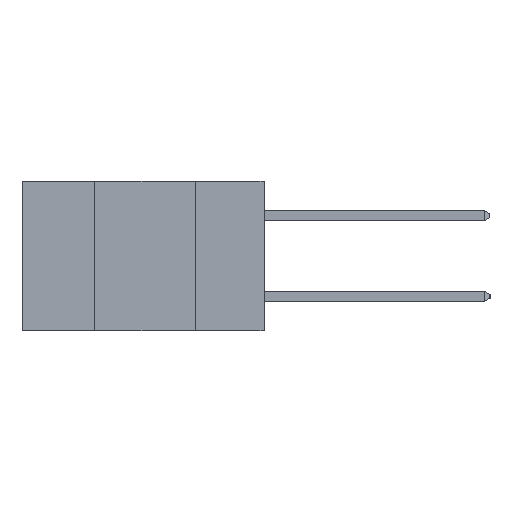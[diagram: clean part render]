
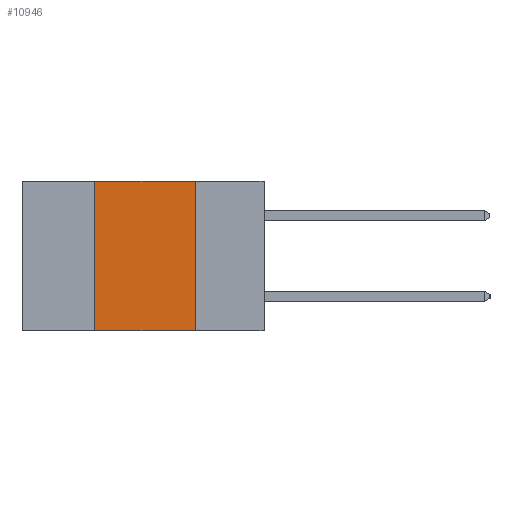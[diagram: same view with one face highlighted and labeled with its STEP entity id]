
A CAD part, left-side view. The second image highlights one B-rep face of the part: STEP entity #10946.
In plain terms, the highlighted planar face has unit normal (-1, 0, 0).
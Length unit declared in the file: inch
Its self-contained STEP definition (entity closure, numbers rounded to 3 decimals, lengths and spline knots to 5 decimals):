
#507 = DIRECTION ( 'NONE',  ( 0., 0., 1. ) ) ;
#640 = CARTESIAN_POINT ( 'NONE',  ( 0., 0.42, -0.37 ) ) ;
#693 = EDGE_CURVE ( 'NONE', #15144, #4478, #11052, .T. ) ;
#1330 = FACE_OUTER_BOUND ( 'NONE', #13095, .T. ) ;
#1433 = DIRECTION ( 'NONE',  ( 0., 0., -1. ) ) ;
#3179 = PLANE ( 'NONE',  #21426 ) ;
#3795 = VECTOR ( 'NONE', #507, 39.37008 ) ;
#4478 = VERTEX_POINT ( 'NONE', #6883 ) ;
#5023 = DIRECTION ( 'NONE',  ( 0., 0., -1. ) ) ;
#5945 = CARTESIAN_POINT ( 'NONE',  ( 0., 0.17, 0. ) ) ;
#6883 = CARTESIAN_POINT ( 'NONE',  ( 0., 0.17, -0.37 ) ) ;
#6891 = CARTESIAN_POINT ( 'NONE',  ( 0., 0.42, 0. ) ) ;
#7694 = EDGE_CURVE ( 'NONE', #15144, #23706, #8826, .T. ) ;
#8826 = LINE ( 'NONE', #640, #3795 ) ;
#9227 = DIRECTION ( 'NONE',  ( 0., -1., 0. ) ) ;
#9640 = LINE ( 'NONE', #14547, #23871 ) ;
#10619 = CARTESIAN_POINT ( 'NONE',  ( 0., 0.6, 0. ) ) ;
#10946 = ADVANCED_FACE ( 'NONE', ( #1330 ), #3179, .F. ) ;
#11052 = LINE ( 'NONE', #21004, #20401 ) ;
#12438 = ORIENTED_EDGE ( 'NONE', *, *, #14450, .F. ) ;
#12713 = DIRECTION ( 'NONE',  ( 0., -1., 0. ) ) ;
#12934 = ORIENTED_EDGE ( 'NONE', *, *, #13826, .F. ) ;
#13095 = EDGE_LOOP ( 'NONE', ( #12438, #12934, #13597, #13920 ) ) ;
#13597 = ORIENTED_EDGE ( 'NONE', *, *, #7694, .F. ) ;
#13826 = EDGE_CURVE ( 'NONE', #23706, #19737, #23029, .T. ) ;
#13920 = ORIENTED_EDGE ( 'NONE', *, *, #693, .T. ) ;
#14450 = EDGE_CURVE ( 'NONE', #19737, #4478, #9640, .T. ) ;
#14547 = CARTESIAN_POINT ( 'NONE',  ( 0., 0.17, -0.37 ) ) ;
#14984 = CARTESIAN_POINT ( 'NONE',  ( 0., 0.6, 0. ) ) ;
#15144 = VERTEX_POINT ( 'NONE', #20185 ) ;
#16277 = DIRECTION ( 'NONE',  ( 1., 0., 0. ) ) ;
#17601 = VECTOR ( 'NONE', #12713, 39.37008 ) ;
#19737 = VERTEX_POINT ( 'NONE', #5945 ) ;
#20185 = CARTESIAN_POINT ( 'NONE',  ( 0., 0.42, -0.37 ) ) ;
#20401 = VECTOR ( 'NONE', #9227, 39.37008 ) ;
#21004 = CARTESIAN_POINT ( 'NONE',  ( 0., 0.6, -0.37 ) ) ;
#21426 = AXIS2_PLACEMENT_3D ( 'NONE', #10619, #16277, #5023 ) ;
#23029 = LINE ( 'NONE', #14984, #17601 ) ;
#23706 = VERTEX_POINT ( 'NONE', #6891 ) ;
#23871 = VECTOR ( 'NONE', #1433, 39.37008 ) ;
